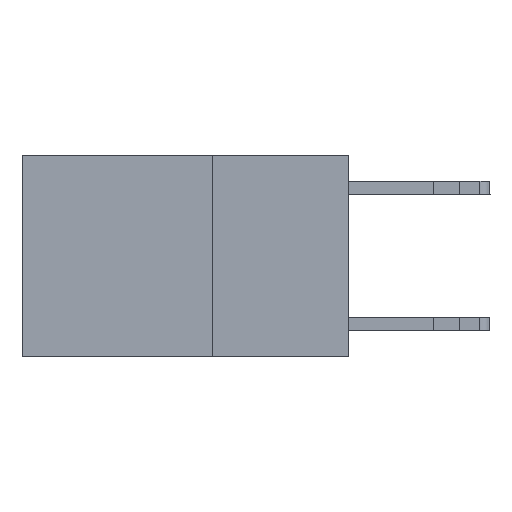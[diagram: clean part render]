
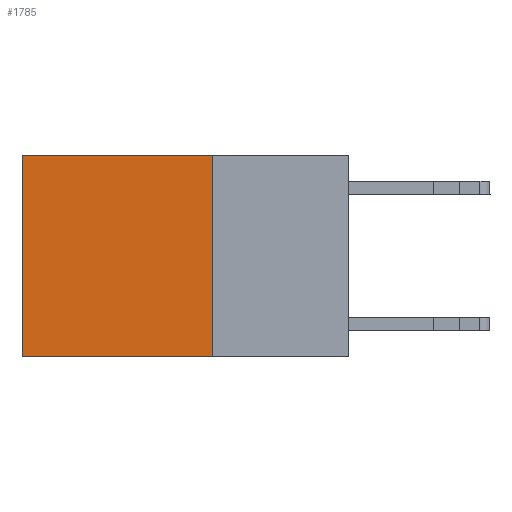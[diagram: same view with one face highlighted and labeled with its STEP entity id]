
A CAD part, left-side view. The second image highlights one B-rep face of the part: STEP entity #1785.
In plain terms, the highlighted planar face has unit normal (-1, 0, 0).
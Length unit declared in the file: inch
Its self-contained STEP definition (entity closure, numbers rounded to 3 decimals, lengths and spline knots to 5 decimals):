
#101 = CARTESIAN_POINT ( 'NONE',  ( 0.2625, 0.25, 0. ) ) ;
#844 = DIRECTION ( 'NONE',  ( 0., 0., -1. ) ) ;
#916 = VERTEX_POINT ( 'NONE', #6354 ) ;
#1129 = ORIENTED_EDGE ( 'NONE', *, *, #11980, .T. ) ;
#1135 = LINE ( 'NONE', #6930, #2547 ) ;
#1640 = VERTEX_POINT ( 'NONE', #2317 ) ;
#1785 = ADVANCED_FACE ( 'NONE', ( #8691 ), #7099, .F. ) ;
#1914 = AXIS2_PLACEMENT_3D ( 'NONE', #4796, #8459, #13212 ) ;
#2317 = CARTESIAN_POINT ( 'NONE',  ( 0.2625, 0.6, -0.37 ) ) ;
#2547 = VECTOR ( 'NONE', #5774, 39.37008 ) ;
#2623 = ORIENTED_EDGE ( 'NONE', *, *, #13684, .T. ) ;
#3194 = CARTESIAN_POINT ( 'NONE',  ( 0.2625, 0.25, -0.37 ) ) ;
#3242 = VECTOR ( 'NONE', #9386, 39.37008 ) ;
#4625 = CARTESIAN_POINT ( 'NONE',  ( 0.2625, 0.25, 0. ) ) ;
#4796 = CARTESIAN_POINT ( 'NONE',  ( 0.2625, 0.25, 0. ) ) ;
#5536 = EDGE_CURVE ( 'NONE', #5558, #1640, #9123, .T. ) ;
#5558 = VERTEX_POINT ( 'NONE', #12717 ) ;
#5774 = DIRECTION ( 'NONE',  ( 0., 0., -1. ) ) ;
#6354 = CARTESIAN_POINT ( 'NONE',  ( 0.2625, 0.6, 0. ) ) ;
#6930 = CARTESIAN_POINT ( 'NONE',  ( 0.2625, 0.6, 0. ) ) ;
#7099 = PLANE ( 'NONE',  #1914 ) ;
#7943 = DIRECTION ( 'NONE',  ( 0., 1., 0. ) ) ;
#8058 = LINE ( 'NONE', #15044, #11023 ) ;
#8459 = DIRECTION ( 'NONE',  ( 1., 0., 0. ) ) ;
#8691 = FACE_OUTER_BOUND ( 'NONE', #14967, .T. ) ;
#8983 = VERTEX_POINT ( 'NONE', #101 ) ;
#9123 = LINE ( 'NONE', #3194, #12101 ) ;
#9386 = DIRECTION ( 'NONE',  ( 0., 1., 0. ) ) ;
#10550 = ORIENTED_EDGE ( 'NONE', *, *, #14523, .F. ) ;
#10557 = LINE ( 'NONE', #4625, #3242 ) ;
#11023 = VECTOR ( 'NONE', #844, 39.37008 ) ;
#11886 = ORIENTED_EDGE ( 'NONE', *, *, #5536, .F. ) ;
#11980 = EDGE_CURVE ( 'NONE', #8983, #916, #10557, .T. ) ;
#12101 = VECTOR ( 'NONE', #7943, 39.37008 ) ;
#12717 = CARTESIAN_POINT ( 'NONE',  ( 0.2625, 0.25, -0.37 ) ) ;
#13212 = DIRECTION ( 'NONE',  ( 0., 0., -1. ) ) ;
#13684 = EDGE_CURVE ( 'NONE', #916, #1640, #1135, .T. ) ;
#14523 = EDGE_CURVE ( 'NONE', #8983, #5558, #8058, .T. ) ;
#14967 = EDGE_LOOP ( 'NONE', ( #2623, #11886, #10550, #1129 ) ) ;
#15044 = CARTESIAN_POINT ( 'NONE',  ( 0.2625, 0.25, 0. ) ) ;
